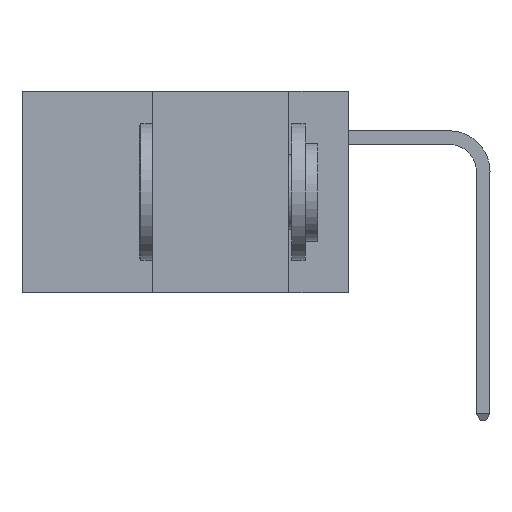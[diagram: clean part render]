
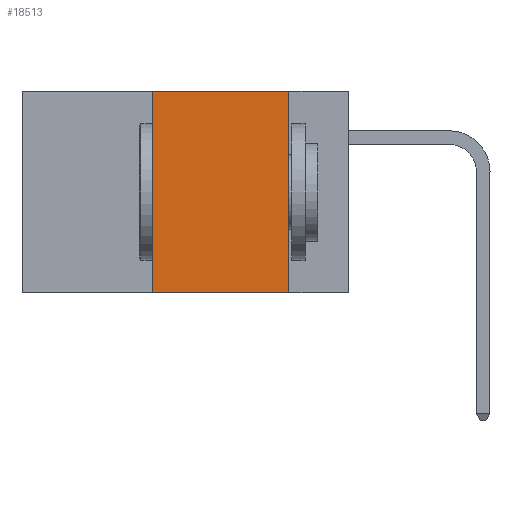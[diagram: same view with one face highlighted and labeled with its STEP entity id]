
A CAD part, left-side view. The second image highlights one B-rep face of the part: STEP entity #18513.
In plain terms, the highlighted planar face has unit normal (-1, 0, 0).
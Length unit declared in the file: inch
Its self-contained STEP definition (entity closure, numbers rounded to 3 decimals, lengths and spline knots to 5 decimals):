
#1193 = LINE ( 'NONE', #11744, #24594 ) ;
#1643 = VERTEX_POINT ( 'NONE', #9774 ) ;
#1990 = CARTESIAN_POINT ( 'NONE',  ( 0., 0.6, 0. ) ) ;
#1994 = ORIENTED_EDGE ( 'NONE', *, *, #22963, .T. ) ;
#2836 = VERTEX_POINT ( 'NONE', #12531 ) ;
#3586 = VERTEX_POINT ( 'NONE', #11072 ) ;
#4766 = AXIS2_PLACEMENT_3D ( 'NONE', #7763, #23658, #28210 ) ;
#4951 = VERTEX_POINT ( 'NONE', #25848 ) ;
#5471 = DIRECTION ( 'NONE',  ( 0., 0., 1. ) ) ;
#6212 = FACE_OUTER_BOUND ( 'NONE', #23725, .T. ) ;
#7651 = CARTESIAN_POINT ( 'NONE',  ( 0., 0.36, 0. ) ) ;
#7763 = CARTESIAN_POINT ( 'NONE',  ( 0., 0.6, 0. ) ) ;
#9451 = DIRECTION ( 'NONE',  ( 0., 0., -1. ) ) ;
#9553 = VECTOR ( 'NONE', #10939, 39.37008 ) ;
#9774 = CARTESIAN_POINT ( 'NONE',  ( 0., 0.11, 0. ) ) ;
#10939 = DIRECTION ( 'NONE',  ( 0., -1., 0. ) ) ;
#11072 = CARTESIAN_POINT ( 'NONE',  ( 0., 0.36, 0. ) ) ;
#11744 = CARTESIAN_POINT ( 'NONE',  ( 0., 0.11, 0. ) ) ;
#11751 = ORIENTED_EDGE ( 'NONE', *, *, #16420, .F. ) ;
#12531 = CARTESIAN_POINT ( 'NONE',  ( 0., 0.11, -0.37 ) ) ;
#12532 = CARTESIAN_POINT ( 'NONE',  ( 0., 0.6, -0.37 ) ) ;
#14892 = DIRECTION ( 'NONE',  ( 0., -1., 0. ) ) ;
#15607 = LINE ( 'NONE', #1990, #9553 ) ;
#15689 = VECTOR ( 'NONE', #14892, 39.37008 ) ;
#16420 = EDGE_CURVE ( 'NONE', #3586, #1643, #15607, .T. ) ;
#16988 = ORIENTED_EDGE ( 'NONE', *, *, #26673, .F. ) ;
#18453 = ORIENTED_EDGE ( 'NONE', *, *, #19810, .F. ) ;
#18513 = ADVANCED_FACE ( 'NONE', ( #6212 ), #21352, .F. ) ;
#19810 = EDGE_CURVE ( 'NONE', #1643, #2836, #1193, .T. ) ;
#21352 = PLANE ( 'NONE',  #4766 ) ;
#22561 = VECTOR ( 'NONE', #5471, 39.37008 ) ;
#22963 = EDGE_CURVE ( 'NONE', #4951, #2836, #26307, .T. ) ;
#23658 = DIRECTION ( 'NONE',  ( 1., 0., 0. ) ) ;
#23725 = EDGE_LOOP ( 'NONE', ( #18453, #11751, #16988, #1994 ) ) ;
#24014 = LINE ( 'NONE', #7651, #22561 ) ;
#24594 = VECTOR ( 'NONE', #9451, 39.37008 ) ;
#25848 = CARTESIAN_POINT ( 'NONE',  ( 0., 0.36, -0.37 ) ) ;
#26307 = LINE ( 'NONE', #12532, #15689 ) ;
#26673 = EDGE_CURVE ( 'NONE', #4951, #3586, #24014, .T. ) ;
#28210 = DIRECTION ( 'NONE',  ( 0., 0., -1. ) ) ;
